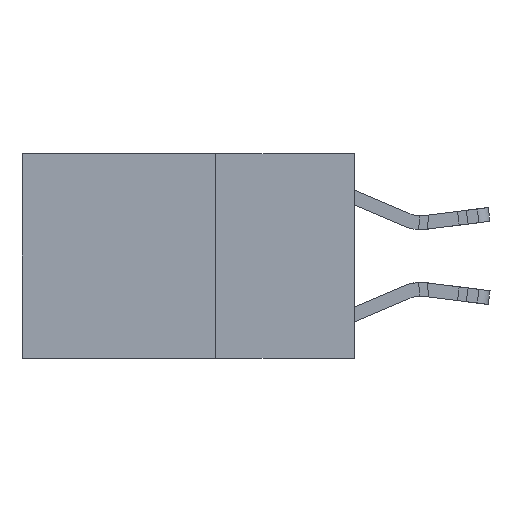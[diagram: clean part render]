
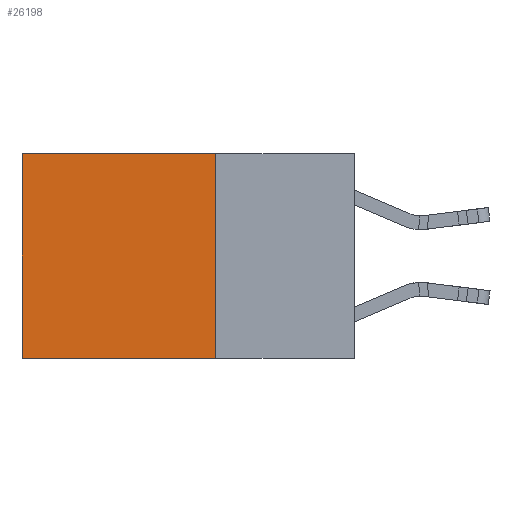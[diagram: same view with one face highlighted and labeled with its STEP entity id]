
A CAD part, left-side view. The second image highlights one B-rep face of the part: STEP entity #26198.
In plain terms, the highlighted planar face has unit normal (-1, 0, 0).
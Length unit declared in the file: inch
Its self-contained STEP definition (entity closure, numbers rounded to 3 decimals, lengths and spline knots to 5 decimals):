
#205 = CARTESIAN_POINT ( 'NONE',  ( 0.2625, 0.25, -0.37 ) ) ;
#520 = DIRECTION ( 'NONE',  ( 0., 0., -1. ) ) ;
#1175 = VECTOR ( 'NONE', #10615, 39.37008 ) ;
#1349 = EDGE_CURVE ( 'NONE', #28902, #28616, #6865, .T. ) ;
#3213 = EDGE_CURVE ( 'NONE', #29768, #28902, #19917, .T. ) ;
#5058 = VECTOR ( 'NONE', #22124, 39.37008 ) ;
#5107 = EDGE_LOOP ( 'NONE', ( #9909, #13964, #28110, #12545 ) ) ;
#5158 = VERTEX_POINT ( 'NONE', #26862 ) ;
#6451 = FACE_OUTER_BOUND ( 'NONE', #5107, .T. ) ;
#6865 = LINE ( 'NONE', #205, #18290 ) ;
#7555 = CARTESIAN_POINT ( 'NONE',  ( 0.2625, 0.6, 0. ) ) ;
#7883 = PLANE ( 'NONE',  #12211 ) ;
#8967 = CARTESIAN_POINT ( 'NONE',  ( 0.2625, 0.25, -0.37 ) ) ;
#9846 = EDGE_CURVE ( 'NONE', #5158, #28616, #22983, .T. ) ;
#9909 = ORIENTED_EDGE ( 'NONE', *, *, #9846, .T. ) ;
#10615 = DIRECTION ( 'NONE',  ( 0., 0., -1. ) ) ;
#12211 = AXIS2_PLACEMENT_3D ( 'NONE', #12783, #15228, #520 ) ;
#12545 = ORIENTED_EDGE ( 'NONE', *, *, #23957, .T. ) ;
#12783 = CARTESIAN_POINT ( 'NONE',  ( 0.2625, 0.25, 0. ) ) ;
#13845 = DIRECTION ( 'NONE',  ( 0., 1., 0. ) ) ;
#13964 = ORIENTED_EDGE ( 'NONE', *, *, #1349, .F. ) ;
#15228 = DIRECTION ( 'NONE',  ( 1., 0., 0. ) ) ;
#17395 = DIRECTION ( 'NONE',  ( 0., 1., 0. ) ) ;
#18290 = VECTOR ( 'NONE', #17395, 39.37008 ) ;
#19917 = LINE ( 'NONE', #25171, #1175 ) ;
#22124 = DIRECTION ( 'NONE',  ( 0., 0., -1. ) ) ;
#22983 = LINE ( 'NONE', #7555, #5058 ) ;
#23294 = VECTOR ( 'NONE', #13845, 39.37008 ) ;
#23957 = EDGE_CURVE ( 'NONE', #29768, #5158, #29711, .T. ) ;
#25171 = CARTESIAN_POINT ( 'NONE',  ( 0.2625, 0.25, 0. ) ) ;
#26198 = ADVANCED_FACE ( 'NONE', ( #6451 ), #7883, .F. ) ;
#26862 = CARTESIAN_POINT ( 'NONE',  ( 0.2625, 0.6, 0. ) ) ;
#28110 = ORIENTED_EDGE ( 'NONE', *, *, #3213, .F. ) ;
#28616 = VERTEX_POINT ( 'NONE', #29325 ) ;
#28902 = VERTEX_POINT ( 'NONE', #8967 ) ;
#29264 = CARTESIAN_POINT ( 'NONE',  ( 0.2625, 0.25, 0. ) ) ;
#29325 = CARTESIAN_POINT ( 'NONE',  ( 0.2625, 0.6, -0.37 ) ) ;
#29711 = LINE ( 'NONE', #30778, #23294 ) ;
#29768 = VERTEX_POINT ( 'NONE', #29264 ) ;
#30778 = CARTESIAN_POINT ( 'NONE',  ( 0.2625, 0.25, 0. ) ) ;
